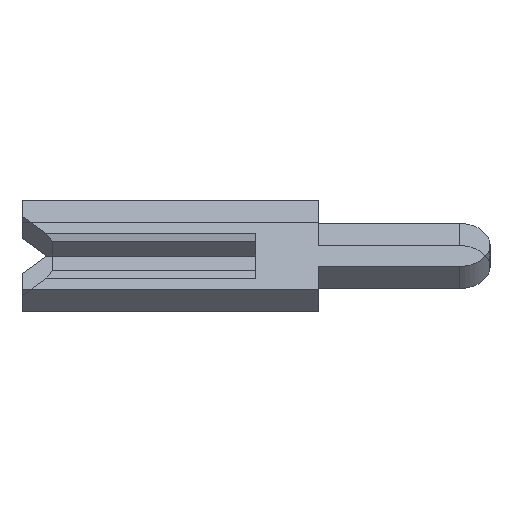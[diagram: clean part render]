
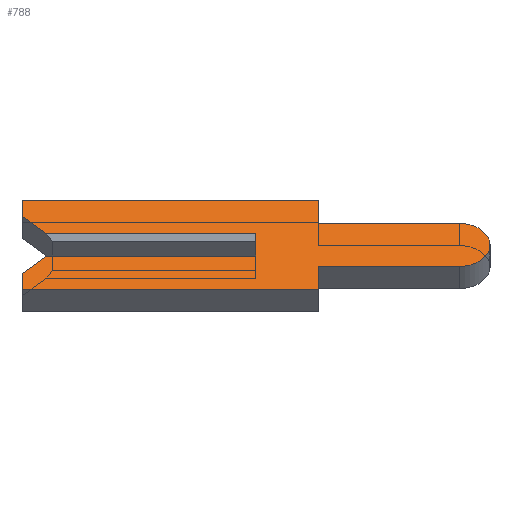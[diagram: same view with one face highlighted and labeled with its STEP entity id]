
A CAD part, left-side view. The second image highlights one B-rep face of the part: STEP entity #788.
In plain terms, the highlighted face is planar.
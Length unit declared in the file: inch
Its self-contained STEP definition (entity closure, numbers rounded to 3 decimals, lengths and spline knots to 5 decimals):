
#33 = CARTESIAN_POINT ( 'NONE',  ( -0.01, 0.15, -0.04 ) ) ;
#79 = CARTESIAN_POINT ( 'NONE',  ( -0.01, 0.15, 0.04 ) ) ;
#105 = CARTESIAN_POINT ( 'NONE',  ( -0.01, 0.15, 0.04 ) ) ;
#107 = VERTEX_POINT ( 'NONE', #1751 ) ;
#130 = CARTESIAN_POINT ( 'NONE',  ( -0.01, 0., -0.01 ) ) ;
#136 = VECTOR ( 'NONE', #1551, 39.37008 ) ;
#151 = VERTEX_POINT ( 'NONE', #258 ) ;
#164 = DIRECTION ( 'NONE',  ( 0., 0., -1. ) ) ;
#194 = AXIS2_PLACEMENT_3D ( 'NONE', #1106, #1437, #1949 ) ;
#235 = DIRECTION ( 'NONE',  ( 0., -1., 0. ) ) ;
#239 = EDGE_CURVE ( 'NONE', #1868, #451, #1142, .T. ) ;
#258 = CARTESIAN_POINT ( 'NONE',  ( -0.01, 0.134, -0.01 ) ) ;
#263 = AXIS2_PLACEMENT_3D ( 'NONE', #1147, #1984, #164 ) ;
#266 = LINE ( 'NONE', #676, #1505 ) ;
#278 = ORIENTED_EDGE ( 'NONE', *, *, #1836, .F. ) ;
#293 = LINE ( 'NONE', #942, #2092 ) ;
#310 = VERTEX_POINT ( 'NONE', #1644 ) ;
#330 = DIRECTION ( 'NONE',  ( 0., -1., 0. ) ) ;
#347 = VECTOR ( 'NONE', #695, 39.37008 ) ;
#368 = CARTESIAN_POINT ( 'NONE',  ( -0.01, 0.15, -0.04 ) ) ;
#388 = EDGE_CURVE ( 'NONE', #548, #760, #1985, .T. ) ;
#428 = VECTOR ( 'NONE', #2052, 39.37008 ) ;
#451 = VERTEX_POINT ( 'NONE', #791 ) ;
#464 = DIRECTION ( 'NONE',  ( 0., 0.707, 0.707 ) ) ;
#466 = EDGE_CURVE ( 'NONE', #310, #107, #579, .T. ) ;
#470 = ORIENTED_EDGE ( 'NONE', *, *, #1916, .F. ) ;
#514 = ORIENTED_EDGE ( 'NONE', *, *, #968, .F. ) ;
#548 = VERTEX_POINT ( 'NONE', #1807 ) ;
#579 = LINE ( 'NONE', #953, #1096 ) ;
#588 = CARTESIAN_POINT ( 'NONE',  ( -0.01, 0.15, 0.026 ) ) ;
#602 = VERTEX_POINT ( 'NONE', #130 ) ;
#618 = EDGE_CURVE ( 'NONE', #451, #856, #293, .T. ) ;
#643 = DIRECTION ( 'NONE',  ( 0., 0., -1. ) ) ;
#672 = ORIENTED_EDGE ( 'NONE', *, *, #1424, .F. ) ;
#676 = CARTESIAN_POINT ( 'NONE',  ( -0.01, 0.1305, -0.0065 ) ) ;
#694 = ORIENTED_EDGE ( 'NONE', *, *, #1084, .F. ) ;
#695 = DIRECTION ( 'NONE',  ( 0., 0., 1. ) ) ;
#708 = ORIENTED_EDGE ( 'NONE', *, *, #239, .F. ) ;
#721 = CARTESIAN_POINT ( 'NONE',  ( -0.01, -0.1305, 0.0195 ) ) ;
#729 = VERTEX_POINT ( 'NONE', #1628 ) ;
#731 = LINE ( 'NONE', #740, #136 ) ;
#740 = CARTESIAN_POINT ( 'NONE',  ( -0.01, -0.04, -0.04 ) ) ;
#752 = ORIENTED_EDGE ( 'NONE', *, *, #1088, .F. ) ;
#760 = VERTEX_POINT ( 'NONE', #1834 ) ;
#761 = ORIENTED_EDGE ( 'NONE', *, *, #618, .F. ) ;
#788 = ADVANCED_FACE ( 'NONE', ( #1662 ), #973, .F. ) ;
#791 = CARTESIAN_POINT ( 'NONE',  ( -0.01, -0.1305, -0.0195 ) ) ;
#834 = CARTESIAN_POINT ( 'NONE',  ( -0.01, -0.04, -0.0195 ) ) ;
#856 = VERTEX_POINT ( 'NONE', #834 ) ;
#857 = CARTESIAN_POINT ( 'NONE',  ( -0.01, -0.04, -0.04 ) ) ;
#940 = EDGE_CURVE ( 'NONE', #310, #1058, #1615, .T. ) ;
#942 = CARTESIAN_POINT ( 'NONE',  ( -0.01, -0.04, -0.0195 ) ) ;
#953 = CARTESIAN_POINT ( 'NONE',  ( -0.01, 0.1305, 0.0065 ) ) ;
#958 = LINE ( 'NONE', #1177, #1800 ) ;
#968 = EDGE_CURVE ( 'NONE', #729, #151, #266, .T. ) ;
#973 = PLANE ( 'NONE',  #263 ) ;
#997 = ORIENTED_EDGE ( 'NONE', *, *, #940, .T. ) ;
#1058 = VERTEX_POINT ( 'NONE', #1839 ) ;
#1065 = LINE ( 'NONE', #368, #1115 ) ;
#1084 = EDGE_CURVE ( 'NONE', #151, #602, #1348, .T. ) ;
#1088 = EDGE_CURVE ( 'NONE', #602, #1058, #958, .T. ) ;
#1096 = VECTOR ( 'NONE', #464, 39.37008 ) ;
#1106 = CARTESIAN_POINT ( 'NONE',  ( -0.01, -0.1305, 0. ) ) ;
#1110 = DIRECTION ( 'NONE',  ( 0., 1., 0. ) ) ;
#1115 = VECTOR ( 'NONE', #1203, 39.37008 ) ;
#1133 = EDGE_LOOP ( 'NONE', ( #997, #752, #694, #514, #1654, #672, #278, #761, #708, #1446, #1711, #1365, #470, #1787 ) ) ;
#1142 = CIRCLE ( 'NONE', #194, 0.0195 ) ;
#1147 = CARTESIAN_POINT ( 'NONE',  ( -0.01, -0.1305, 0. ) ) ;
#1177 = CARTESIAN_POINT ( 'NONE',  ( -0.01, 0., 0.0065 ) ) ;
#1203 = DIRECTION ( 'NONE',  ( 0., 1., 0. ) ) ;
#1210 = EDGE_CURVE ( 'NONE', #1362, #729, #1249, .T. ) ;
#1221 = LINE ( 'NONE', #588, #1773 ) ;
#1249 = LINE ( 'NONE', #1378, #347 ) ;
#1271 = VECTOR ( 'NONE', #235, 39.37008 ) ;
#1274 = VECTOR ( 'NONE', #1316, 39.37008 ) ;
#1296 = VECTOR ( 'NONE', #330, 39.37008 ) ;
#1316 = DIRECTION ( 'NONE',  ( 0., -1., 0. ) ) ;
#1348 = LINE ( 'NONE', #1474, #1274 ) ;
#1362 = VERTEX_POINT ( 'NONE', #33 ) ;
#1365 = ORIENTED_EDGE ( 'NONE', *, *, #1820, .F. ) ;
#1378 = CARTESIAN_POINT ( 'NONE',  ( -0.01, 0.15, -0.026 ) ) ;
#1424 = EDGE_CURVE ( 'NONE', #1465, #1362, #1065, .T. ) ;
#1437 = DIRECTION ( 'NONE',  ( 1., 0., 0. ) ) ;
#1446 = ORIENTED_EDGE ( 'NONE', *, *, #1726, .F. ) ;
#1465 = VERTEX_POINT ( 'NONE', #857 ) ;
#1474 = CARTESIAN_POINT ( 'NONE',  ( -0.01, -0.1305, -0.01 ) ) ;
#1505 = VECTOR ( 'NONE', #1830, 39.37008 ) ;
#1551 = DIRECTION ( 'NONE',  ( 0., 0., -1. ) ) ;
#1557 = LINE ( 'NONE', #79, #428 ) ;
#1615 = LINE ( 'NONE', #1649, #1296 ) ;
#1628 = CARTESIAN_POINT ( 'NONE',  ( -0.01, 0.15, -0.026 ) ) ;
#1644 = CARTESIAN_POINT ( 'NONE',  ( -0.01, 0.134, 0.01 ) ) ;
#1649 = CARTESIAN_POINT ( 'NONE',  ( -0.01, 0.15, 0.01 ) ) ;
#1654 = ORIENTED_EDGE ( 'NONE', *, *, #1210, .F. ) ;
#1659 = DIRECTION ( 'NONE',  ( 0., 0., 1. ) ) ;
#1662 = FACE_OUTER_BOUND ( 'NONE', #1133, .T. ) ;
#1685 = VECTOR ( 'NONE', #643, 39.37008 ) ;
#1711 = ORIENTED_EDGE ( 'NONE', *, *, #388, .F. ) ;
#1726 = EDGE_CURVE ( 'NONE', #760, #1868, #1744, .T. ) ;
#1735 = CARTESIAN_POINT ( 'NONE',  ( -0.01, -0.04, 0.0195 ) ) ;
#1744 = LINE ( 'NONE', #1735, #1271 ) ;
#1751 = CARTESIAN_POINT ( 'NONE',  ( -0.01, 0.15, 0.026 ) ) ;
#1773 = VECTOR ( 'NONE', #1891, 39.37008 ) ;
#1787 = ORIENTED_EDGE ( 'NONE', *, *, #466, .F. ) ;
#1800 = VECTOR ( 'NONE', #1659, 39.37008 ) ;
#1807 = CARTESIAN_POINT ( 'NONE',  ( -0.01, -0.04, 0.04 ) ) ;
#1820 = EDGE_CURVE ( 'NONE', #1919, #548, #1557, .T. ) ;
#1830 = DIRECTION ( 'NONE',  ( 0., -0.707, 0.707 ) ) ;
#1834 = CARTESIAN_POINT ( 'NONE',  ( -0.01, -0.04, 0.0195 ) ) ;
#1836 = EDGE_CURVE ( 'NONE', #856, #1465, #731, .T. ) ;
#1839 = CARTESIAN_POINT ( 'NONE',  ( -0.01, 0., 0.01 ) ) ;
#1868 = VERTEX_POINT ( 'NONE', #721 ) ;
#1891 = DIRECTION ( 'NONE',  ( 0., 0., 1. ) ) ;
#1916 = EDGE_CURVE ( 'NONE', #107, #1919, #1221, .T. ) ;
#1919 = VERTEX_POINT ( 'NONE', #105 ) ;
#1949 = DIRECTION ( 'NONE',  ( 0., 0., -1. ) ) ;
#1972 = CARTESIAN_POINT ( 'NONE',  ( -0.01, -0.04, 0.04 ) ) ;
#1984 = DIRECTION ( 'NONE',  ( 1., 0., 0. ) ) ;
#1985 = LINE ( 'NONE', #1972, #1685 ) ;
#2052 = DIRECTION ( 'NONE',  ( 0., -1., 0. ) ) ;
#2092 = VECTOR ( 'NONE', #1110, 39.37008 ) ;
